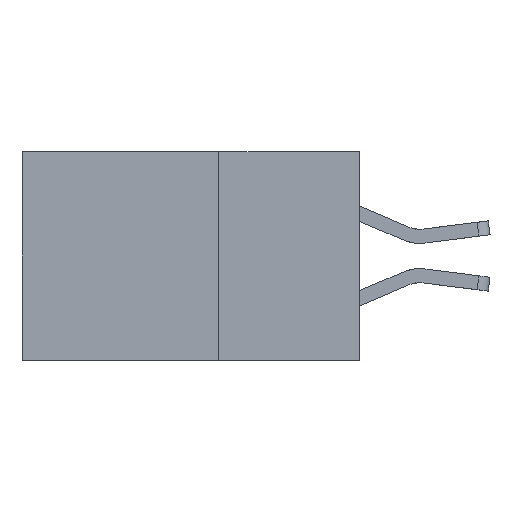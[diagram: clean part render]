
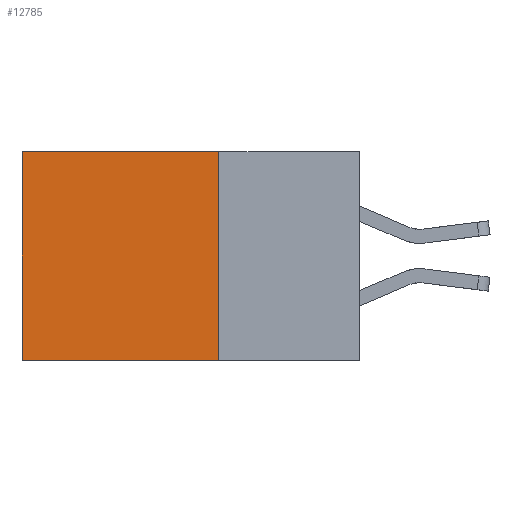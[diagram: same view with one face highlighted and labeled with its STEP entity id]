
A CAD part, left-side view. The second image highlights one B-rep face of the part: STEP entity #12785.
In plain terms, the highlighted planar face has unit normal (-1, 0, 0).
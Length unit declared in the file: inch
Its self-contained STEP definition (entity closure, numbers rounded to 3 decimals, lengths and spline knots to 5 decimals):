
#807 = CARTESIAN_POINT ( 'NONE',  ( 0.2875, 0.6, -0.37 ) ) ;
#1472 = DIRECTION ( 'NONE',  ( 0., 1., 0. ) ) ;
#2180 = CARTESIAN_POINT ( 'NONE',  ( 0.2875, 0.6, 0. ) ) ;
#3004 = VERTEX_POINT ( 'NONE', #807 ) ;
#3745 = PLANE ( 'NONE',  #11158 ) ;
#4211 = CARTESIAN_POINT ( 'NONE',  ( 0.2875, 0.25, 0. ) ) ;
#4399 = DIRECTION ( 'NONE',  ( 0., 0., -1. ) ) ;
#4617 = EDGE_LOOP ( 'NONE', ( #11699, #12132, #12819, #14540 ) ) ;
#4901 = CARTESIAN_POINT ( 'NONE',  ( 0.2875, 0.25, 0. ) ) ;
#5047 = LINE ( 'NONE', #9617, #14130 ) ;
#5102 = VECTOR ( 'NONE', #8576, 39.37008 ) ;
#5753 = FACE_OUTER_BOUND ( 'NONE', #4617, .T. ) ;
#6041 = DIRECTION ( 'NONE',  ( 0., 0., -1. ) ) ;
#6042 = VERTEX_POINT ( 'NONE', #13325 ) ;
#7379 = EDGE_CURVE ( 'NONE', #10843, #3004, #11038, .T. ) ;
#8576 = DIRECTION ( 'NONE',  ( 0., 1., 0. ) ) ;
#9617 = CARTESIAN_POINT ( 'NONE',  ( 0.2875, 0.25, 0. ) ) ;
#10102 = CARTESIAN_POINT ( 'NONE',  ( 0.2875, 0.6, 0. ) ) ;
#10791 = CARTESIAN_POINT ( 'NONE',  ( 0.2875, 0.25, -0.37 ) ) ;
#10843 = VERTEX_POINT ( 'NONE', #2180 ) ;
#11038 = LINE ( 'NONE', #10102, #14422 ) ;
#11085 = EDGE_CURVE ( 'NONE', #12298, #3004, #11506, .T. ) ;
#11158 = AXIS2_PLACEMENT_3D ( 'NONE', #4901, #12842, #6041 ) ;
#11271 = LINE ( 'NONE', #4211, #13938 ) ;
#11506 = LINE ( 'NONE', #11898, #5102 ) ;
#11699 = ORIENTED_EDGE ( 'NONE', *, *, #7379, .T. ) ;
#11898 = CARTESIAN_POINT ( 'NONE',  ( 0.2875, 0.25, -0.37 ) ) ;
#12132 = ORIENTED_EDGE ( 'NONE', *, *, #11085, .F. ) ;
#12298 = VERTEX_POINT ( 'NONE', #10791 ) ;
#12785 = ADVANCED_FACE ( 'NONE', ( #5753 ), #3745, .F. ) ;
#12819 = ORIENTED_EDGE ( 'NONE', *, *, #13026, .F. ) ;
#12842 = DIRECTION ( 'NONE',  ( 1., 0., 0. ) ) ;
#12857 = EDGE_CURVE ( 'NONE', #6042, #10843, #5047, .T. ) ;
#13026 = EDGE_CURVE ( 'NONE', #6042, #12298, #11271, .T. ) ;
#13299 = DIRECTION ( 'NONE',  ( 0., 0., -1. ) ) ;
#13325 = CARTESIAN_POINT ( 'NONE',  ( 0.2875, 0.25, 0. ) ) ;
#13938 = VECTOR ( 'NONE', #13299, 39.37008 ) ;
#14130 = VECTOR ( 'NONE', #1472, 39.37008 ) ;
#14422 = VECTOR ( 'NONE', #4399, 39.37008 ) ;
#14540 = ORIENTED_EDGE ( 'NONE', *, *, #12857, .T. ) ;
